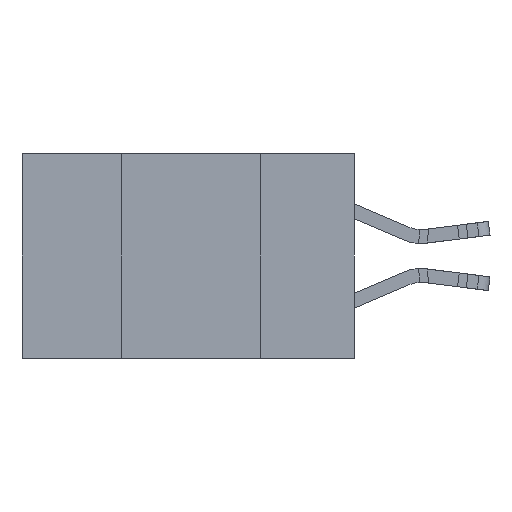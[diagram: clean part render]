
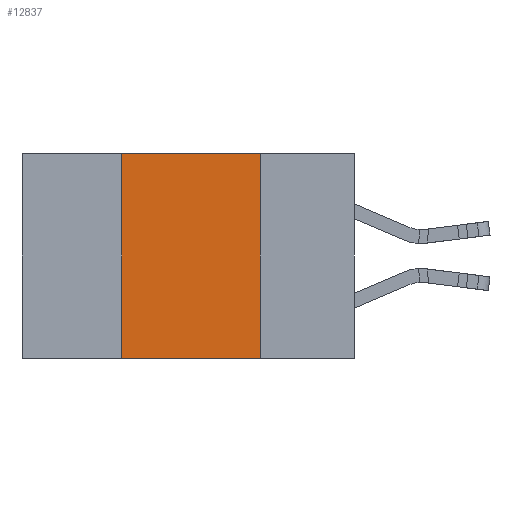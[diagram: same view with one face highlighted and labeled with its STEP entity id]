
A CAD part, left-side view. The second image highlights one B-rep face of the part: STEP entity #12837.
In plain terms, the highlighted planar face has unit normal (-1, 0, 0).
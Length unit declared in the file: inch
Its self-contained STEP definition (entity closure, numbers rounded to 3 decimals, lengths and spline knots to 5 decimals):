
#492 = EDGE_CURVE ( 'NONE', #6475, #12612, #24028, .T. ) ;
#542 = CARTESIAN_POINT ( 'NONE',  ( 0., 0.6, -0.37 ) ) ;
#1219 = ORIENTED_EDGE ( 'NONE', *, *, #29199, .F. ) ;
#1518 = DIRECTION ( 'NONE',  ( 0., -1., 0. ) ) ;
#3589 = VERTEX_POINT ( 'NONE', #10647 ) ;
#3952 = VECTOR ( 'NONE', #6765, 39.37008 ) ;
#4130 = CARTESIAN_POINT ( 'NONE',  ( 0., 0.6, 0. ) ) ;
#5915 = CARTESIAN_POINT ( 'NONE',  ( 0., 0.42, 0. ) ) ;
#6475 = VERTEX_POINT ( 'NONE', #17668 ) ;
#6765 = DIRECTION ( 'NONE',  ( 0., 0., 1. ) ) ;
#7234 = EDGE_LOOP ( 'NONE', ( #32024, #1219, #10993, #18699 ) ) ;
#9713 = DIRECTION ( 'NONE',  ( 0., 0., -1. ) ) ;
#10153 = FACE_OUTER_BOUND ( 'NONE', #7234, .T. ) ;
#10647 = CARTESIAN_POINT ( 'NONE',  ( 0., 0.17, -0.37 ) ) ;
#10690 = VECTOR ( 'NONE', #1518, 39.37008 ) ;
#10696 = AXIS2_PLACEMENT_3D ( 'NONE', #4130, #29229, #14309 ) ;
#10993 = ORIENTED_EDGE ( 'NONE', *, *, #492, .F. ) ;
#11793 = PLANE ( 'NONE',  #10696 ) ;
#12612 = VERTEX_POINT ( 'NONE', #5915 ) ;
#12837 = ADVANCED_FACE ( 'NONE', ( #10153 ), #11793, .F. ) ;
#13569 = VERTEX_POINT ( 'NONE', #32112 ) ;
#14309 = DIRECTION ( 'NONE',  ( 0., 0., -1. ) ) ;
#15474 = LINE ( 'NONE', #542, #27919 ) ;
#15628 = EDGE_CURVE ( 'NONE', #13569, #3589, #24446, .T. ) ;
#15805 = LINE ( 'NONE', #16627, #10690 ) ;
#16627 = CARTESIAN_POINT ( 'NONE',  ( 0., 0.6, 0. ) ) ;
#17668 = CARTESIAN_POINT ( 'NONE',  ( 0., 0.42, -0.37 ) ) ;
#18699 = ORIENTED_EDGE ( 'NONE', *, *, #27033, .T. ) ;
#20672 = DIRECTION ( 'NONE',  ( 0., -1., 0. ) ) ;
#24028 = LINE ( 'NONE', #29390, #3952 ) ;
#24446 = LINE ( 'NONE', #24702, #31017 ) ;
#24702 = CARTESIAN_POINT ( 'NONE',  ( 0., 0.17, 0. ) ) ;
#27033 = EDGE_CURVE ( 'NONE', #6475, #3589, #15474, .T. ) ;
#27919 = VECTOR ( 'NONE', #20672, 39.37008 ) ;
#29199 = EDGE_CURVE ( 'NONE', #12612, #13569, #15805, .T. ) ;
#29229 = DIRECTION ( 'NONE',  ( 1., 0., 0. ) ) ;
#29390 = CARTESIAN_POINT ( 'NONE',  ( 0., 0.42, 0. ) ) ;
#31017 = VECTOR ( 'NONE', #9713, 39.37008 ) ;
#32024 = ORIENTED_EDGE ( 'NONE', *, *, #15628, .F. ) ;
#32112 = CARTESIAN_POINT ( 'NONE',  ( 0., 0.17, 0. ) ) ;
